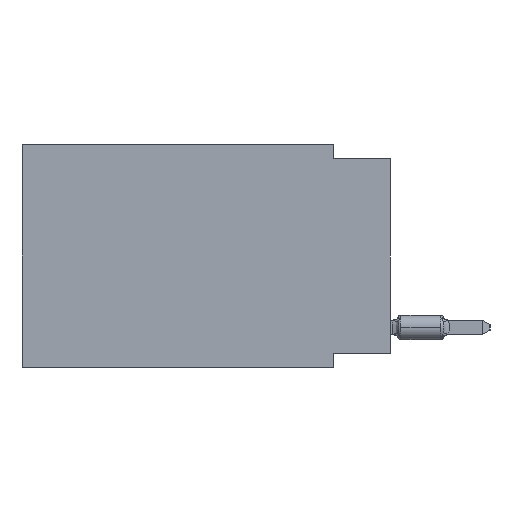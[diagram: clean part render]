
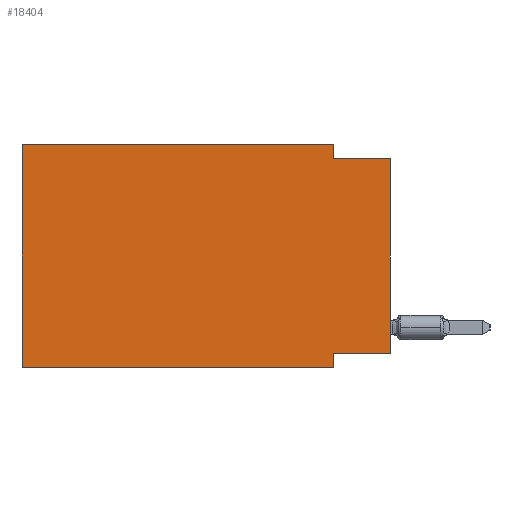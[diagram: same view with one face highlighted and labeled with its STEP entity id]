
A CAD part, left-side view. The second image highlights one B-rep face of the part: STEP entity #18404.
In plain terms, the highlighted planar face has unit normal (-1, 0, 0).
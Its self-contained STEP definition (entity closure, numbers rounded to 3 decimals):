
#53 = EDGE_CURVE ( 'NONE', #6004, #4388, #580, .T. ) ;
#261 = CARTESIAN_POINT ( 'NONE',  ( 0., 2.54, -9.906 ) ) ;
#580 = LINE ( 'NONE', #19892, #24408 ) ;
#624 = ORIENTED_EDGE ( 'NONE', *, *, #21629, .F. ) ;
#991 = VECTOR ( 'NONE', #4477, 1000. ) ;
#1777 = VECTOR ( 'NONE', #20104, 1000. ) ;
#2055 = VERTEX_POINT ( 'NONE', #11969 ) ;
#2205 = CARTESIAN_POINT ( 'NONE',  ( 0., 16.383, 0. ) ) ;
#2855 = DIRECTION ( 'NONE',  ( 0., 1., 0. ) ) ;
#3300 = LINE ( 'NONE', #15130, #23003 ) ;
#3592 = ORIENTED_EDGE ( 'NONE', *, *, #53, .F. ) ;
#4338 = CARTESIAN_POINT ( 'NONE',  ( 0., 0., 0. ) ) ;
#4388 = VERTEX_POINT ( 'NONE', #11964 ) ;
#4454 = LINE ( 'NONE', #24161, #1777 ) ;
#4477 = DIRECTION ( 'NONE',  ( 0., -1., 0. ) ) ;
#5220 = ORIENTED_EDGE ( 'NONE', *, *, #23053, .T. ) ;
#5414 = CARTESIAN_POINT ( 'NONE',  ( 0., 2.54, -9.906 ) ) ;
#6004 = VERTEX_POINT ( 'NONE', #10043 ) ;
#6232 = ORIENTED_EDGE ( 'NONE', *, *, #6789, .F. ) ;
#6683 = EDGE_LOOP ( 'NONE', ( #5220, #11082, #24668, #6232, #3592, #8186, #18871, #624 ) ) ;
#6789 = EDGE_CURVE ( 'NONE', #4388, #16522, #9858, .T. ) ;
#7141 = CARTESIAN_POINT ( 'NONE',  ( 0., 2.54, -0.635 ) ) ;
#8186 = ORIENTED_EDGE ( 'NONE', *, *, #9608, .T. ) ;
#8356 = DIRECTION ( 'NONE',  ( 0., 0., -1. ) ) ;
#8678 = VECTOR ( 'NONE', #22737, 1000. ) ;
#8734 = DIRECTION ( 'NONE',  ( 1., 0., 0. ) ) ;
#8956 = CARTESIAN_POINT ( 'NONE',  ( 0., 0., -9.271 ) ) ;
#9283 = LINE ( 'NONE', #20856, #8678 ) ;
#9608 = EDGE_CURVE ( 'NONE', #6004, #20677, #3300, .T. ) ;
#9858 = LINE ( 'NONE', #2205, #991 ) ;
#10043 = CARTESIAN_POINT ( 'NONE',  ( 0., 16.383, -9.906 ) ) ;
#10629 = LINE ( 'NONE', #23691, #17963 ) ;
#10793 = FACE_OUTER_BOUND ( 'NONE', #6683, .T. ) ;
#11082 = ORIENTED_EDGE ( 'NONE', *, *, #23123, .F. ) ;
#11738 = AXIS2_PLACEMENT_3D ( 'NONE', #14091, #8734, #8356 ) ;
#11913 = VERTEX_POINT ( 'NONE', #8956 ) ;
#11964 = CARTESIAN_POINT ( 'NONE',  ( 0., 16.383, 0. ) ) ;
#11969 = CARTESIAN_POINT ( 'NONE',  ( 0., 0., -0.635 ) ) ;
#12284 = VERTEX_POINT ( 'NONE', #14778 ) ;
#12736 = CARTESIAN_POINT ( 'NONE',  ( 0., 2.54, 0. ) ) ;
#14062 = EDGE_CURVE ( 'NONE', #16522, #16653, #9283, .T. ) ;
#14091 = CARTESIAN_POINT ( 'NONE',  ( 0., 16.383, 0. ) ) ;
#14778 = CARTESIAN_POINT ( 'NONE',  ( 0., 2.54, -9.271 ) ) ;
#15130 = CARTESIAN_POINT ( 'NONE',  ( 0., 16.383, -9.906 ) ) ;
#16522 = VERTEX_POINT ( 'NONE', #12736 ) ;
#16653 = VERTEX_POINT ( 'NONE', #7141 ) ;
#16975 = VECTOR ( 'NONE', #24856, 1000. ) ;
#17362 = EDGE_CURVE ( 'NONE', #12284, #20677, #20555, .T. ) ;
#17963 = VECTOR ( 'NONE', #2855, 1000. ) ;
#18074 = DIRECTION ( 'NONE',  ( 0., 0., 1. ) ) ;
#18404 = ADVANCED_FACE ( 'NONE', ( #10793 ), #23722, .F. ) ;
#18871 = ORIENTED_EDGE ( 'NONE', *, *, #17362, .F. ) ;
#19525 = DIRECTION ( 'NONE',  ( 0., 0., 1. ) ) ;
#19623 = VECTOR ( 'NONE', #18074, 1000. ) ;
#19892 = CARTESIAN_POINT ( 'NONE',  ( 0., 16.383, 0. ) ) ;
#20104 = DIRECTION ( 'NONE',  ( 0., -1., 0. ) ) ;
#20555 = LINE ( 'NONE', #5414, #16975 ) ;
#20677 = VERTEX_POINT ( 'NONE', #261 ) ;
#20856 = CARTESIAN_POINT ( 'NONE',  ( 0., 2.54, 0. ) ) ;
#21629 = EDGE_CURVE ( 'NONE', #11913, #12284, #10629, .T. ) ;
#21754 = LINE ( 'NONE', #4338, #19623 ) ;
#22737 = DIRECTION ( 'NONE',  ( 0., 0., -1. ) ) ;
#23003 = VECTOR ( 'NONE', #25026, 1000. ) ;
#23053 = EDGE_CURVE ( 'NONE', #11913, #2055, #21754, .T. ) ;
#23123 = EDGE_CURVE ( 'NONE', #16653, #2055, #4454, .T. ) ;
#23691 = CARTESIAN_POINT ( 'NONE',  ( 0., 0., -9.271 ) ) ;
#23722 = PLANE ( 'NONE',  #11738 ) ;
#24161 = CARTESIAN_POINT ( 'NONE',  ( 0., 0., -0.635 ) ) ;
#24408 = VECTOR ( 'NONE', #19525, 1000. ) ;
#24668 = ORIENTED_EDGE ( 'NONE', *, *, #14062, .F. ) ;
#24856 = DIRECTION ( 'NONE',  ( 0., 0., -1. ) ) ;
#25026 = DIRECTION ( 'NONE',  ( 0., -1., 0. ) ) ;
